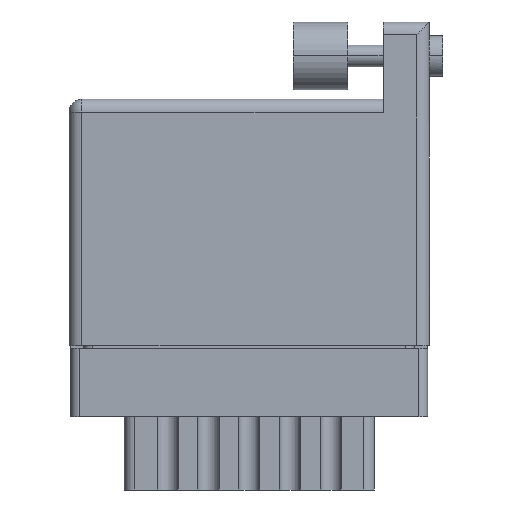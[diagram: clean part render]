
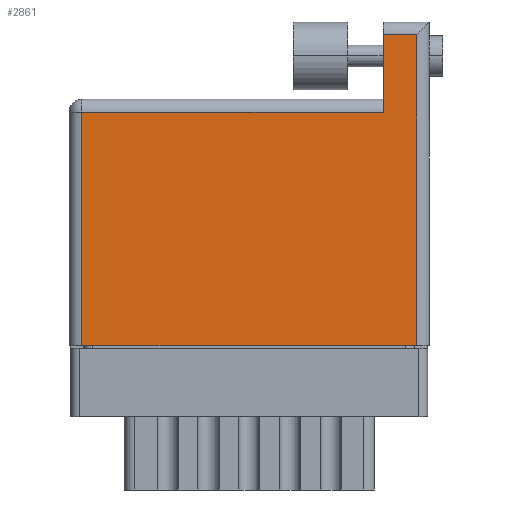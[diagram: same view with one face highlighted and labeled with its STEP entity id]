
A CAD part, front view. The second image highlights one B-rep face of the part: STEP entity #2861.
In plain terms, the highlighted face is planar.
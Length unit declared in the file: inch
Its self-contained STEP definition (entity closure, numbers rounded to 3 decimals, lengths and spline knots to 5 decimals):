
#194 = VECTOR ( 'NONE', #27092, 39.37008 ) ;
#215 = CARTESIAN_POINT ( 'NONE',  ( 1.155, 0.859, 0. ) ) ;
#418 = DIRECTION ( 'NONE',  ( -1., 0., 0. ) ) ;
#681 = CARTESIAN_POINT ( 'NONE',  ( 0.047, 0., 0. ) ) ;
#1016 = VERTEX_POINT ( 'NONE', #24585 ) ;
#1180 = EDGE_CURVE ( 'NONE', #5032, #25088, #17211, .T. ) ;
#1815 = DIRECTION ( 'NONE',  ( 0., 0., -1. ) ) ;
#2144 = EDGE_CURVE ( 'NONE', #22860, #1016, #29330, .T. ) ;
#2861 = ADVANCED_FACE ( 'NONE', ( #27496 ), #18365, .F. ) ;
#3973 = VECTOR ( 'NONE', #13619, 39.37008 ) ;
#4480 = CARTESIAN_POINT ( 'NONE',  ( 0., 0.906, 0. ) ) ;
#4693 = DIRECTION ( 'NONE',  ( -1., 0., 0. ) ) ;
#4891 = DIRECTION ( 'NONE',  ( 1., 0., 0. ) ) ;
#4931 = CARTESIAN_POINT ( 'NONE',  ( 0.047, 0., 0. ) ) ;
#5032 = VERTEX_POINT ( 'NONE', #21230 ) ;
#5171 = LINE ( 'NONE', #4931, #25413 ) ;
#7851 = CARTESIAN_POINT ( 'NONE',  ( 0., 0.859, 0. ) ) ;
#8808 = ORIENTED_EDGE ( 'NONE', *, *, #2144, .T. ) ;
#9342 = LINE ( 'NONE', #23689, #17067 ) ;
#9403 = CARTESIAN_POINT ( 'NONE',  ( 1.278, 0., 0. ) ) ;
#9646 = CARTESIAN_POINT ( 'NONE',  ( 1.155, 1.143, 0. ) ) ;
#10397 = EDGE_CURVE ( 'NONE', #14915, #22860, #9342, .T. ) ;
#10855 = AXIS2_PLACEMENT_3D ( 'NONE', #4480, #1815, #4693 ) ;
#11289 = LINE ( 'NONE', #7851, #23422 ) ;
#11532 = EDGE_LOOP ( 'NONE', ( #22276, #8808, #12736, #29485, #18552, #25086 ) ) ;
#12736 = ORIENTED_EDGE ( 'NONE', *, *, #15727, .T. ) ;
#13619 = DIRECTION ( 'NONE',  ( 0., -1., 0. ) ) ;
#14915 = VERTEX_POINT ( 'NONE', #681 ) ;
#15549 = CARTESIAN_POINT ( 'NONE',  ( 1.278, 1.19, 0. ) ) ;
#15640 = LINE ( 'NONE', #9646, #22990 ) ;
#15727 = EDGE_CURVE ( 'NONE', #1016, #5032, #15640, .T. ) ;
#17067 = VECTOR ( 'NONE', #4891, 39.37008 ) ;
#17211 = LINE ( 'NONE', #30271, #3973 ) ;
#18365 = PLANE ( 'NONE',  #10855 ) ;
#18552 = ORIENTED_EDGE ( 'NONE', *, *, #20635, .T. ) ;
#20233 = VERTEX_POINT ( 'NONE', #21020 ) ;
#20635 = EDGE_CURVE ( 'NONE', #25088, #20233, #11289, .T. ) ;
#21020 = CARTESIAN_POINT ( 'NONE',  ( 0.047, 0.859, 0. ) ) ;
#21230 = CARTESIAN_POINT ( 'NONE',  ( 1.155, 1.143, 0. ) ) ;
#22276 = ORIENTED_EDGE ( 'NONE', *, *, #10397, .T. ) ;
#22860 = VERTEX_POINT ( 'NONE', #9403 ) ;
#22990 = VECTOR ( 'NONE', #418, 39.37008 ) ;
#23422 = VECTOR ( 'NONE', #24290, 39.37008 ) ;
#23689 = CARTESIAN_POINT ( 'NONE',  ( 0., 0., 0. ) ) ;
#24290 = DIRECTION ( 'NONE',  ( -1., 0., 0. ) ) ;
#24585 = CARTESIAN_POINT ( 'NONE',  ( 1.278, 1.143, 0. ) ) ;
#25086 = ORIENTED_EDGE ( 'NONE', *, *, #28273, .T. ) ;
#25088 = VERTEX_POINT ( 'NONE', #215 ) ;
#25413 = VECTOR ( 'NONE', #25596, 39.37008 ) ;
#25596 = DIRECTION ( 'NONE',  ( 0., -1., 0. ) ) ;
#27092 = DIRECTION ( 'NONE',  ( 0., 1., 0. ) ) ;
#27496 = FACE_OUTER_BOUND ( 'NONE', #11532, .T. ) ;
#28273 = EDGE_CURVE ( 'NONE', #20233, #14915, #5171, .T. ) ;
#29330 = LINE ( 'NONE', #15549, #194 ) ;
#29485 = ORIENTED_EDGE ( 'NONE', *, *, #1180, .T. ) ;
#30271 = CARTESIAN_POINT ( 'NONE',  ( 1.155, 1.19, 0. ) ) ;
